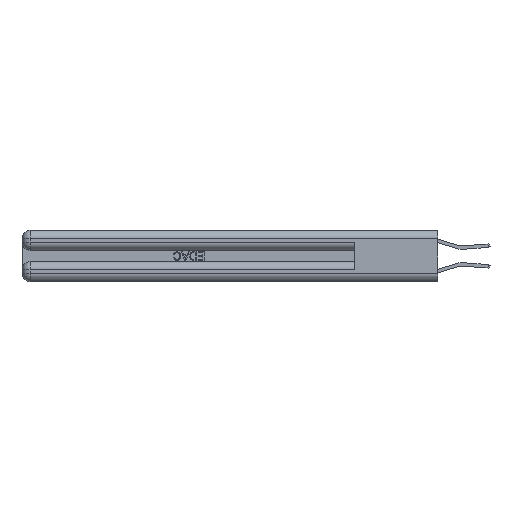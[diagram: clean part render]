
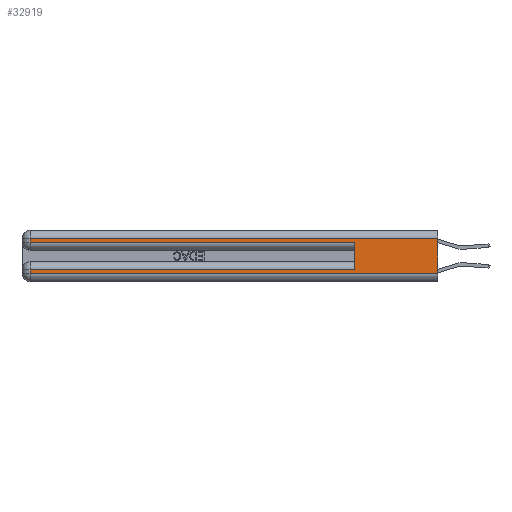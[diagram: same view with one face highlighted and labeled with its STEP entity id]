
A CAD part, left-side view. The second image highlights one B-rep face of the part: STEP entity #32919.
In plain terms, the highlighted planar face has unit normal (-1, 0, 0).
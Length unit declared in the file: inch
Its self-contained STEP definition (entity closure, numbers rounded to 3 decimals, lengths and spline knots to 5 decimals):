
#1321 = EDGE_CURVE ( 'NONE', #7704, #31762, #32263, .T. ) ;
#1391 = CARTESIAN_POINT ( 'NONE',  ( 0., 0., 0.285 ) ) ;
#1572 = CARTESIAN_POINT ( 'NONE',  ( 0., 2.94, 0.37 ) ) ;
#1639 = DIRECTION ( 'NONE',  ( 0., 0., -1. ) ) ;
#1714 = VERTEX_POINT ( 'NONE', #13083 ) ;
#2417 = CARTESIAN_POINT ( 'NONE',  ( 0., 0., 0.085 ) ) ;
#2423 = VECTOR ( 'NONE', #4197, 39.37008 ) ;
#2563 = CARTESIAN_POINT ( 'NONE',  ( 0., 2.94, 0.31 ) ) ;
#3001 = CARTESIAN_POINT ( 'NONE',  ( 0., 0., 0.31 ) ) ;
#3208 = ORIENTED_EDGE ( 'NONE', *, *, #30515, .T. ) ;
#3871 = EDGE_CURVE ( 'NONE', #20886, #15838, #13347, .T. ) ;
#4197 = DIRECTION ( 'NONE',  ( 0., -1., 0. ) ) ;
#4654 = EDGE_CURVE ( 'NONE', #18111, #31762, #25382, .T. ) ;
#4685 = VECTOR ( 'NONE', #23968, 39.37008 ) ;
#4867 = LINE ( 'NONE', #2417, #22952 ) ;
#7033 = DIRECTION ( 'NONE',  ( 1., 0., 0. ) ) ;
#7135 = ORIENTED_EDGE ( 'NONE', *, *, #17261, .T. ) ;
#7320 = DIRECTION ( 'NONE',  ( 0., 0., -1. ) ) ;
#7704 = VERTEX_POINT ( 'NONE', #22743 ) ;
#8620 = EDGE_CURVE ( 'NONE', #15838, #18111, #20021, .T. ) ;
#8769 = ORIENTED_EDGE ( 'NONE', *, *, #3871, .T. ) ;
#9677 = PLANE ( 'NONE',  #29603 ) ;
#11073 = DIRECTION ( 'NONE',  ( 0., 1., 0. ) ) ;
#11835 = ORIENTED_EDGE ( 'NONE', *, *, #4654, .T. ) ;
#12926 = VECTOR ( 'NONE', #15403, 39.37008 ) ;
#13083 = CARTESIAN_POINT ( 'NONE',  ( 0., 2.94, 0.06 ) ) ;
#13284 = LINE ( 'NONE', #29408, #24075 ) ;
#13299 = CARTESIAN_POINT ( 'NONE',  ( 0., 0.6, 0.145 ) ) ;
#13347 = LINE ( 'NONE', #3001, #28685 ) ;
#14394 = ORIENTED_EDGE ( 'NONE', *, *, #17943, .F. ) ;
#15095 = DIRECTION ( 'NONE',  ( 0., 0., -1. ) ) ;
#15255 = ORIENTED_EDGE ( 'NONE', *, *, #8620, .T. ) ;
#15403 = DIRECTION ( 'NONE',  ( 0., 0., -1. ) ) ;
#15838 = VERTEX_POINT ( 'NONE', #2563 ) ;
#17261 = EDGE_CURVE ( 'NONE', #17872, #1714, #20825, .T. ) ;
#17872 = VERTEX_POINT ( 'NONE', #18032 ) ;
#17943 = EDGE_CURVE ( 'NONE', #20886, #26372, #30881, .T. ) ;
#18032 = CARTESIAN_POINT ( 'NONE',  ( 0., 2.94, 0.085 ) ) ;
#18111 = VERTEX_POINT ( 'NONE', #18202 ) ;
#18202 = CARTESIAN_POINT ( 'NONE',  ( 0., 2.94, 0.285 ) ) ;
#19664 = FACE_OUTER_BOUND ( 'NONE', #24126, .T. ) ;
#20021 = LINE ( 'NONE', #30763, #28438 ) ;
#20348 = CARTESIAN_POINT ( 'NONE',  ( 0., 0., 0.37 ) ) ;
#20825 = LINE ( 'NONE', #1572, #29437 ) ;
#20886 = VERTEX_POINT ( 'NONE', #24212 ) ;
#20988 = DIRECTION ( 'NONE',  ( 0., 1., 0. ) ) ;
#22743 = CARTESIAN_POINT ( 'NONE',  ( 0., 0.6, 0.085 ) ) ;
#22952 = VECTOR ( 'NONE', #20988, 39.37008 ) ;
#23968 = DIRECTION ( 'NONE',  ( 0., 0., 1. ) ) ;
#24075 = VECTOR ( 'NONE', #34208, 39.37008 ) ;
#24126 = EDGE_LOOP ( 'NONE', ( #14394, #8769, #15255, #11835, #31375, #3208, #7135, #29116 ) ) ;
#24212 = CARTESIAN_POINT ( 'NONE',  ( 0., 0., 0.31 ) ) ;
#25382 = LINE ( 'NONE', #1391, #2423 ) ;
#25391 = CARTESIAN_POINT ( 'NONE',  ( 0., 0., 0.37 ) ) ;
#26372 = VERTEX_POINT ( 'NONE', #28674 ) ;
#28438 = VECTOR ( 'NONE', #1639, 39.37008 ) ;
#28674 = CARTESIAN_POINT ( 'NONE',  ( 0., 0., 0.06 ) ) ;
#28685 = VECTOR ( 'NONE', #11073, 39.37008 ) ;
#29116 = ORIENTED_EDGE ( 'NONE', *, *, #30568, .T. ) ;
#29408 = CARTESIAN_POINT ( 'NONE',  ( 0., 0., 0.06 ) ) ;
#29437 = VECTOR ( 'NONE', #7320, 39.37008 ) ;
#29603 = AXIS2_PLACEMENT_3D ( 'NONE', #20348, #7033, #15095 ) ;
#30515 = EDGE_CURVE ( 'NONE', #7704, #17872, #4867, .T. ) ;
#30568 = EDGE_CURVE ( 'NONE', #1714, #26372, #13284, .T. ) ;
#30763 = CARTESIAN_POINT ( 'NONE',  ( 0., 2.94, 0.37 ) ) ;
#30881 = LINE ( 'NONE', #25391, #12926 ) ;
#31375 = ORIENTED_EDGE ( 'NONE', *, *, #1321, .F. ) ;
#31762 = VERTEX_POINT ( 'NONE', #32254 ) ;
#32254 = CARTESIAN_POINT ( 'NONE',  ( 0., 0.6, 0.285 ) ) ;
#32263 = LINE ( 'NONE', #13299, #4685 ) ;
#32919 = ADVANCED_FACE ( 'NONE', ( #19664 ), #9677, .F. ) ;
#34208 = DIRECTION ( 'NONE',  ( 0., -1., 0. ) ) ;
